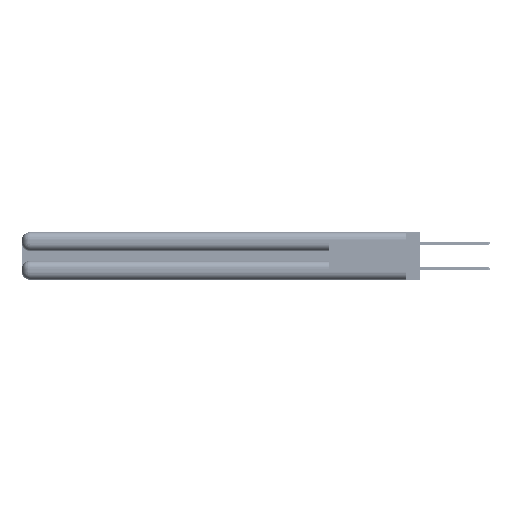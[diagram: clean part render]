
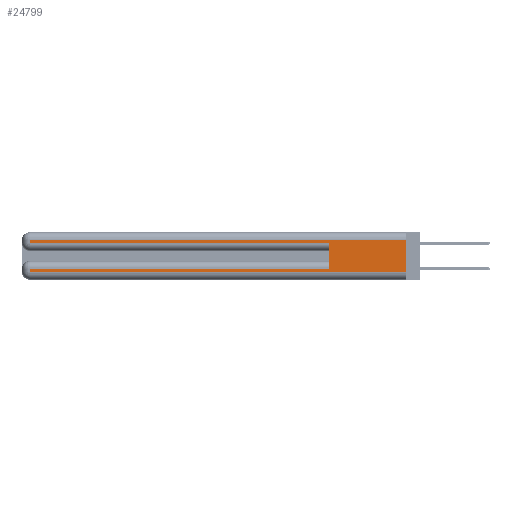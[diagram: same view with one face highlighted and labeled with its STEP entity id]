
A CAD part, left-side view. The second image highlights one B-rep face of the part: STEP entity #24799.
In plain terms, the highlighted planar face has unit normal (-1, 0, 0).
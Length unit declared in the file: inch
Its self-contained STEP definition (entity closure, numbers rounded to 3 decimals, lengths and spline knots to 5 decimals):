
#555 = CARTESIAN_POINT ( 'NONE',  ( 0., 0.6, 0.085 ) ) ;
#700 = VERTEX_POINT ( 'NONE', #555 ) ;
#1027 = EDGE_CURVE ( 'NONE', #6300, #16307, #7896, .T. ) ;
#1621 = ORIENTED_EDGE ( 'NONE', *, *, #41639, .T. ) ;
#4875 = EDGE_CURVE ( 'NONE', #700, #11855, #48777, .T. ) ;
#5673 = CARTESIAN_POINT ( 'NONE',  ( 0., 2.94, 0.31 ) ) ;
#6300 = VERTEX_POINT ( 'NONE', #50483 ) ;
#6840 = ORIENTED_EDGE ( 'NONE', *, *, #13891, .F. ) ;
#7896 = LINE ( 'NONE', #44762, #47438 ) ;
#11673 = LINE ( 'NONE', #41140, #50584 ) ;
#11855 = VERTEX_POINT ( 'NONE', #45198 ) ;
#12062 = EDGE_CURVE ( 'NONE', #13445, #6300, #27571, .T. ) ;
#12877 = DIRECTION ( 'NONE',  ( 1., 0., 0. ) ) ;
#13445 = VERTEX_POINT ( 'NONE', #19636 ) ;
#13485 = LINE ( 'NONE', #14762, #17874 ) ;
#13549 = CARTESIAN_POINT ( 'NONE',  ( 0., 2.94, 0.285 ) ) ;
#13891 = EDGE_CURVE ( 'NONE', #23778, #16307, #47412, .T. ) ;
#13935 = DIRECTION ( 'NONE',  ( 0., 0., -1. ) ) ;
#14762 = CARTESIAN_POINT ( 'NONE',  ( 0., 0., 0.285 ) ) ;
#16121 = EDGE_CURVE ( 'NONE', #23778, #40118, #11673, .T. ) ;
#16307 = VERTEX_POINT ( 'NONE', #30121 ) ;
#16431 = VECTOR ( 'NONE', #34239, 39.37008 ) ;
#16886 = EDGE_CURVE ( 'NONE', #38563, #11855, #13485, .T. ) ;
#17175 = DIRECTION ( 'NONE',  ( 0., 0., 1. ) ) ;
#17352 = CARTESIAN_POINT ( 'NONE',  ( 0., 0.6, 0.145 ) ) ;
#17874 = VECTOR ( 'NONE', #46823, 39.37008 ) ;
#19636 = CARTESIAN_POINT ( 'NONE',  ( 0., 2.94, 0.085 ) ) ;
#23778 = VERTEX_POINT ( 'NONE', #38258 ) ;
#24525 = ORIENTED_EDGE ( 'NONE', *, *, #12062, .T. ) ;
#24564 = AXIS2_PLACEMENT_3D ( 'NONE', #29768, #12877, #13935 ) ;
#24604 = ORIENTED_EDGE ( 'NONE', *, *, #4875, .F. ) ;
#24799 = ADVANCED_FACE ( 'NONE', ( #34936 ), #29953, .F. ) ;
#25566 = CARTESIAN_POINT ( 'NONE',  ( 0., 2.94, 0.37 ) ) ;
#25957 = CARTESIAN_POINT ( 'NONE',  ( 0., 0., 0.085 ) ) ;
#26269 = CARTESIAN_POINT ( 'NONE',  ( 0., 0., 0.37 ) ) ;
#27081 = ORIENTED_EDGE ( 'NONE', *, *, #1027, .T. ) ;
#27571 = LINE ( 'NONE', #25566, #28178 ) ;
#27993 = VECTOR ( 'NONE', #50628, 39.37008 ) ;
#28178 = VECTOR ( 'NONE', #30679, 39.37008 ) ;
#29768 = CARTESIAN_POINT ( 'NONE',  ( 0., 0., 0.37 ) ) ;
#29953 = PLANE ( 'NONE',  #24564 ) ;
#30121 = CARTESIAN_POINT ( 'NONE',  ( 0., 0., 0.06 ) ) ;
#30679 = DIRECTION ( 'NONE',  ( 0., 0., -1. ) ) ;
#31340 = ORIENTED_EDGE ( 'NONE', *, *, #16121, .T. ) ;
#32955 = VECTOR ( 'NONE', #46122, 39.37008 ) ;
#33450 = LINE ( 'NONE', #46766, #16431 ) ;
#34239 = DIRECTION ( 'NONE',  ( 0., 0., -1. ) ) ;
#34936 = FACE_OUTER_BOUND ( 'NONE', #51963, .T. ) ;
#35239 = ORIENTED_EDGE ( 'NONE', *, *, #16886, .T. ) ;
#38258 = CARTESIAN_POINT ( 'NONE',  ( 0., 0., 0.31 ) ) ;
#38563 = VERTEX_POINT ( 'NONE', #13549 ) ;
#39210 = LINE ( 'NONE', #25957, #32955 ) ;
#40017 = VECTOR ( 'NONE', #17175, 39.37008 ) ;
#40118 = VERTEX_POINT ( 'NONE', #5673 ) ;
#40720 = DIRECTION ( 'NONE',  ( 0., -1., 0. ) ) ;
#41140 = CARTESIAN_POINT ( 'NONE',  ( 0., 0., 0.31 ) ) ;
#41639 = EDGE_CURVE ( 'NONE', #700, #13445, #39210, .T. ) ;
#41819 = DIRECTION ( 'NONE',  ( 0., 1., 0. ) ) ;
#43499 = ORIENTED_EDGE ( 'NONE', *, *, #48727, .T. ) ;
#44762 = CARTESIAN_POINT ( 'NONE',  ( 0., 0., 0.06 ) ) ;
#45198 = CARTESIAN_POINT ( 'NONE',  ( 0., 0.6, 0.285 ) ) ;
#46122 = DIRECTION ( 'NONE',  ( 0., 1., 0. ) ) ;
#46766 = CARTESIAN_POINT ( 'NONE',  ( 0., 2.94, 0.37 ) ) ;
#46823 = DIRECTION ( 'NONE',  ( 0., -1., 0. ) ) ;
#47412 = LINE ( 'NONE', #26269, #27993 ) ;
#47438 = VECTOR ( 'NONE', #40720, 39.37008 ) ;
#48727 = EDGE_CURVE ( 'NONE', #40118, #38563, #33450, .T. ) ;
#48777 = LINE ( 'NONE', #17352, #40017 ) ;
#50483 = CARTESIAN_POINT ( 'NONE',  ( 0., 2.94, 0.06 ) ) ;
#50584 = VECTOR ( 'NONE', #41819, 39.37008 ) ;
#50628 = DIRECTION ( 'NONE',  ( 0., 0., -1. ) ) ;
#51963 = EDGE_LOOP ( 'NONE', ( #6840, #31340, #43499, #35239, #24604, #1621, #24525, #27081 ) ) ;
